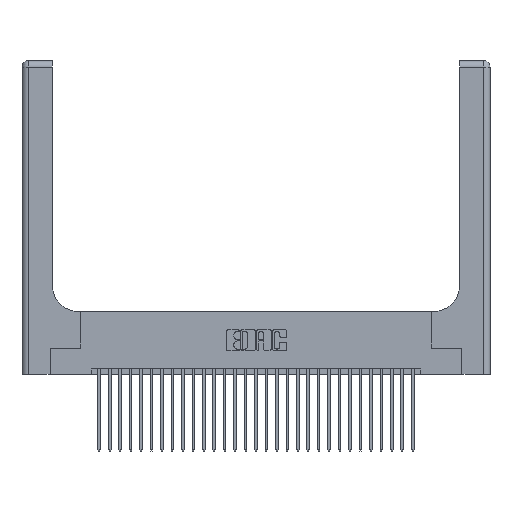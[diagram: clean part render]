
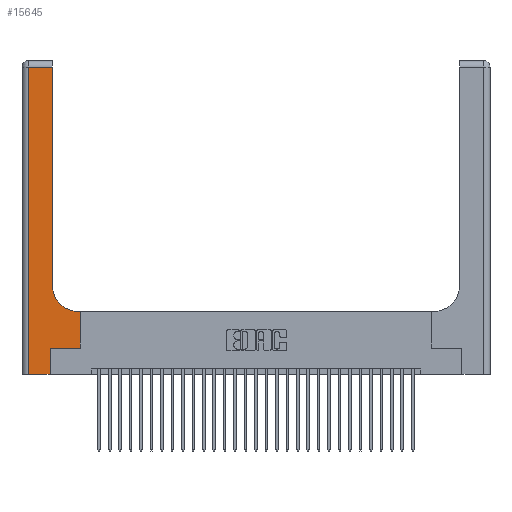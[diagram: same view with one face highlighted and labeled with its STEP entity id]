
A CAD part, top view. The second image highlights one B-rep face of the part: STEP entity #15645.
In plain terms, the highlighted planar face has unit normal (0, 0, 1).
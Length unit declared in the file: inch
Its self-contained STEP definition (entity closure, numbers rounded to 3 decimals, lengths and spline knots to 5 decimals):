
#40 = EDGE_CURVE ( 'NONE', #27251, #1459, #28681, .T. ) ;
#75 = VERTEX_POINT ( 'NONE', #25451 ) ;
#257 = LINE ( 'NONE', #28040, #29854 ) ;
#321 = EDGE_CURVE ( 'NONE', #13569, #6173, #3624, .T. ) ;
#847 = EDGE_CURVE ( 'NONE', #75, #10420, #26746, .T. ) ;
#1061 = VERTEX_POINT ( 'NONE', #29521 ) ;
#1459 = VERTEX_POINT ( 'NONE', #21840 ) ;
#1542 = VERTEX_POINT ( 'NONE', #5420 ) ;
#1979 = EDGE_LOOP ( 'NONE', ( #11428, #7515, #25055, #15708, #10439, #17941, #14690, #24704, #21467 ) ) ;
#2621 = CARTESIAN_POINT ( 'NONE',  ( 0.2915, 0.85, 0.37 ) ) ;
#3301 = CARTESIAN_POINT ( 'NONE',  ( 0.06, 2.94, 0.37 ) ) ;
#3624 = LINE ( 'NONE', #14431, #21973 ) ;
#4387 = CARTESIAN_POINT ( 'NONE',  ( 0.269, 0.25, 0.37 ) ) ;
#4640 = EDGE_CURVE ( 'NONE', #16865, #13569, #10951, .T. ) ;
#4948 = LINE ( 'NONE', #29952, #16961 ) ;
#5420 = CARTESIAN_POINT ( 'NONE',  ( 0.269, 0.25, 0.37 ) ) ;
#5855 = FACE_OUTER_BOUND ( 'NONE', #1979, .T. ) ;
#6173 = VERTEX_POINT ( 'NONE', #29144 ) ;
#6675 = DIRECTION ( 'NONE',  ( 0., 1., 0. ) ) ;
#6737 = VECTOR ( 'NONE', #20119, 39.37008 ) ;
#7305 = DIRECTION ( 'NONE',  ( -1., 0., 0. ) ) ;
#7507 = CARTESIAN_POINT ( 'NONE',  ( 0.5415, 0.85, 0.37 ) ) ;
#7515 = ORIENTED_EDGE ( 'NONE', *, *, #12405, .T. ) ;
#8975 = LINE ( 'NONE', #29620, #6737 ) ;
#9624 = PLANE ( 'NONE',  #26080 ) ;
#9682 = VECTOR ( 'NONE', #30102, 39.37008 ) ;
#9935 = DIRECTION ( 'NONE',  ( 1., 0., 0. ) ) ;
#10420 = VERTEX_POINT ( 'NONE', #16004 ) ;
#10439 = ORIENTED_EDGE ( 'NONE', *, *, #13313, .T. ) ;
#10879 = EDGE_CURVE ( 'NONE', #1459, #1061, #4948, .T. ) ;
#10951 = CIRCLE ( 'NONE', #27385, 0.25 ) ;
#11428 = ORIENTED_EDGE ( 'NONE', *, *, #321, .T. ) ;
#11883 = DIRECTION ( 'NONE',  ( 0., 1., 0. ) ) ;
#12405 = EDGE_CURVE ( 'NONE', #6173, #27251, #8975, .T. ) ;
#13313 = EDGE_CURVE ( 'NONE', #1061, #1542, #257, .T. ) ;
#13569 = VERTEX_POINT ( 'NONE', #2621 ) ;
#14431 = CARTESIAN_POINT ( 'NONE',  ( 0.2915, 3., 0.37 ) ) ;
#14451 = CARTESIAN_POINT ( 'NONE',  ( 0., 3., 0.37 ) ) ;
#14690 = ORIENTED_EDGE ( 'NONE', *, *, #847, .T. ) ;
#15486 = EDGE_CURVE ( 'NONE', #1542, #75, #28644, .T. ) ;
#15645 = ADVANCED_FACE ( 'NONE', ( #5855 ), #9624, .F. ) ;
#15708 = ORIENTED_EDGE ( 'NONE', *, *, #10879, .T. ) ;
#15775 = DIRECTION ( 'NONE',  ( 1., 0., 0. ) ) ;
#16004 = CARTESIAN_POINT ( 'NONE',  ( 0.5585, 0.6, 0.37 ) ) ;
#16542 = LINE ( 'NONE', #27116, #27663 ) ;
#16760 = VECTOR ( 'NONE', #21119, 39.37008 ) ;
#16865 = VERTEX_POINT ( 'NONE', #19511 ) ;
#16961 = VECTOR ( 'NONE', #15775, 39.37008 ) ;
#17941 = ORIENTED_EDGE ( 'NONE', *, *, #15486, .T. ) ;
#19511 = CARTESIAN_POINT ( 'NONE',  ( 0.5415, 0.6, 0.37 ) ) ;
#20103 = DIRECTION ( 'NONE',  ( -1., 0., 0. ) ) ;
#20119 = DIRECTION ( 'NONE',  ( -1., 0., 0. ) ) ;
#20466 = VECTOR ( 'NONE', #11883, 39.37008 ) ;
#21119 = DIRECTION ( 'NONE',  ( 1., 0., 0. ) ) ;
#21467 = ORIENTED_EDGE ( 'NONE', *, *, #4640, .T. ) ;
#21502 = DIRECTION ( 'NONE',  ( 0., 1., 0. ) ) ;
#21624 = DIRECTION ( 'NONE',  ( 0., 0., -1. ) ) ;
#21840 = CARTESIAN_POINT ( 'NONE',  ( 0.06, 0., 0.37 ) ) ;
#21973 = VECTOR ( 'NONE', #21502, 39.37008 ) ;
#24231 = DIRECTION ( 'NONE',  ( 0., 0., -1. ) ) ;
#24704 = ORIENTED_EDGE ( 'NONE', *, *, #26866, .T. ) ;
#25055 = ORIENTED_EDGE ( 'NONE', *, *, #40, .T. ) ;
#25348 = CARTESIAN_POINT ( 'NONE',  ( 0.06, 3., 0.37 ) ) ;
#25451 = CARTESIAN_POINT ( 'NONE',  ( 0.5585, 0.25, 0.37 ) ) ;
#26080 = AXIS2_PLACEMENT_3D ( 'NONE', #14451, #21624, #7305 ) ;
#26138 = CARTESIAN_POINT ( 'NONE',  ( 0.5585, 0.25, 0.37 ) ) ;
#26746 = LINE ( 'NONE', #26138, #20466 ) ;
#26866 = EDGE_CURVE ( 'NONE', #10420, #16865, #16542, .T. ) ;
#27116 = CARTESIAN_POINT ( 'NONE',  ( 0.2915, 0.6, 0.37 ) ) ;
#27251 = VERTEX_POINT ( 'NONE', #3301 ) ;
#27385 = AXIS2_PLACEMENT_3D ( 'NONE', #7507, #24231, #9935 ) ;
#27663 = VECTOR ( 'NONE', #20103, 39.37008 ) ;
#28040 = CARTESIAN_POINT ( 'NONE',  ( 0.269, 0., 0.37 ) ) ;
#28644 = LINE ( 'NONE', #4387, #16760 ) ;
#28681 = LINE ( 'NONE', #25348, #9682 ) ;
#29144 = CARTESIAN_POINT ( 'NONE',  ( 0.2915, 2.94, 0.37 ) ) ;
#29521 = CARTESIAN_POINT ( 'NONE',  ( 0.269, 0., 0.37 ) ) ;
#29620 = CARTESIAN_POINT ( 'NONE',  ( 0., 2.94, 0.37 ) ) ;
#29854 = VECTOR ( 'NONE', #6675, 39.37008 ) ;
#29952 = CARTESIAN_POINT ( 'NONE',  ( 0., 0., 0.37 ) ) ;
#30102 = DIRECTION ( 'NONE',  ( 0., -1., 0. ) ) ;
